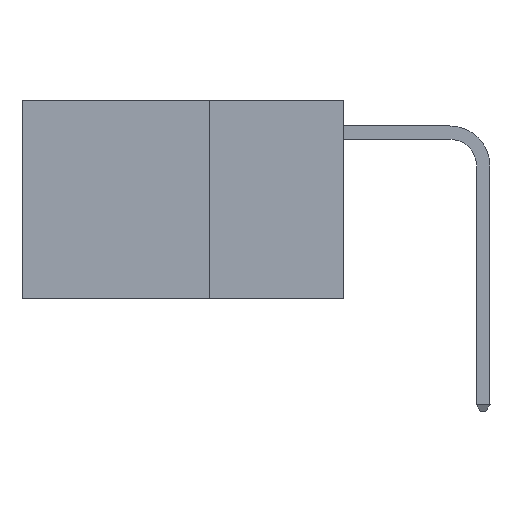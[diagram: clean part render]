
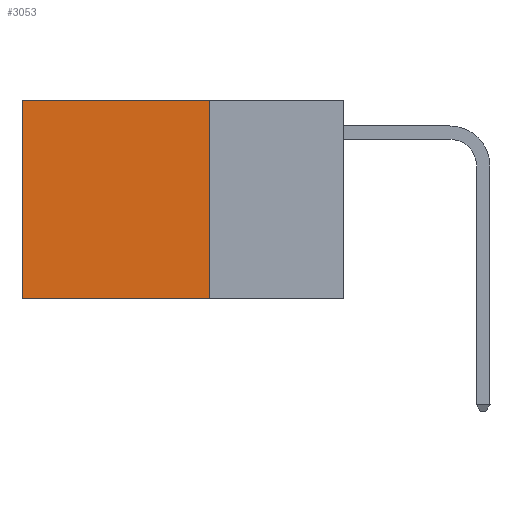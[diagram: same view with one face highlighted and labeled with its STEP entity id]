
A CAD part, left-side view. The second image highlights one B-rep face of the part: STEP entity #3053.
In plain terms, the highlighted planar face has unit normal (-1, 0, 0).
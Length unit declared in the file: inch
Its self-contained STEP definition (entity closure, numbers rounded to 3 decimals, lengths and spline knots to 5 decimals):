
#1074 = ORIENTED_EDGE ( 'NONE', *, *, #3014, .T. ) ;
#3014 = EDGE_CURVE ( 'NONE', #25161, #12816, #27019, .T. ) ;
#3053 = ADVANCED_FACE ( 'NONE', ( #16735 ), #4203, .F. ) ;
#3682 = CARTESIAN_POINT ( 'NONE',  ( 0.2625, 0.25, -0.37 ) ) ;
#3978 = LINE ( 'NONE', #10493, #15912 ) ;
#4203 = PLANE ( 'NONE',  #10961 ) ;
#6119 = ORIENTED_EDGE ( 'NONE', *, *, #11628, .F. ) ;
#6129 = DIRECTION ( 'NONE',  ( 1., 0., 0. ) ) ;
#8317 = VECTOR ( 'NONE', #14834, 39.37008 ) ;
#9080 = ORIENTED_EDGE ( 'NONE', *, *, #14601, .T. ) ;
#9186 = EDGE_LOOP ( 'NONE', ( #9080, #6119, #14605, #1074 ) ) ;
#10493 = CARTESIAN_POINT ( 'NONE',  ( 0.2625, 0.6, 0. ) ) ;
#10961 = AXIS2_PLACEMENT_3D ( 'NONE', #12627, #6129, #22755 ) ;
#11268 = LINE ( 'NONE', #19592, #15796 ) ;
#11628 = EDGE_CURVE ( 'NONE', #15929, #20287, #11268, .T. ) ;
#12627 = CARTESIAN_POINT ( 'NONE',  ( 0.2625, 0.25, 0. ) ) ;
#12816 = VERTEX_POINT ( 'NONE', #13556 ) ;
#13047 = CARTESIAN_POINT ( 'NONE',  ( 0.2625, 0.6, -0.37 ) ) ;
#13556 = CARTESIAN_POINT ( 'NONE',  ( 0.2625, 0.6, 0. ) ) ;
#14308 = EDGE_CURVE ( 'NONE', #25161, #15929, #25434, .T. ) ;
#14601 = EDGE_CURVE ( 'NONE', #12816, #20287, #3978, .T. ) ;
#14605 = ORIENTED_EDGE ( 'NONE', *, *, #14308, .F. ) ;
#14834 = DIRECTION ( 'NONE',  ( 0., 1., 0. ) ) ;
#14988 = DIRECTION ( 'NONE',  ( 0., 1., 0. ) ) ;
#15796 = VECTOR ( 'NONE', #14988, 39.37008 ) ;
#15912 = VECTOR ( 'NONE', #24595, 39.37008 ) ;
#15929 = VERTEX_POINT ( 'NONE', #3682 ) ;
#16735 = FACE_OUTER_BOUND ( 'NONE', #9186, .T. ) ;
#19133 = DIRECTION ( 'NONE',  ( 0., 0., -1. ) ) ;
#19592 = CARTESIAN_POINT ( 'NONE',  ( 0.2625, 0.25, -0.37 ) ) ;
#20287 = VERTEX_POINT ( 'NONE', #13047 ) ;
#21547 = VECTOR ( 'NONE', #19133, 39.37008 ) ;
#22755 = DIRECTION ( 'NONE',  ( 0., 0., -1. ) ) ;
#23034 = CARTESIAN_POINT ( 'NONE',  ( 0.2625, 0.25, 0. ) ) ;
#24595 = DIRECTION ( 'NONE',  ( 0., 0., -1. ) ) ;
#25161 = VERTEX_POINT ( 'NONE', #23034 ) ;
#25304 = CARTESIAN_POINT ( 'NONE',  ( 0.2625, 0.25, 0. ) ) ;
#25361 = CARTESIAN_POINT ( 'NONE',  ( 0.2625, 0.25, 0. ) ) ;
#25434 = LINE ( 'NONE', #25304, #21547 ) ;
#27019 = LINE ( 'NONE', #25361, #8317 ) ;
